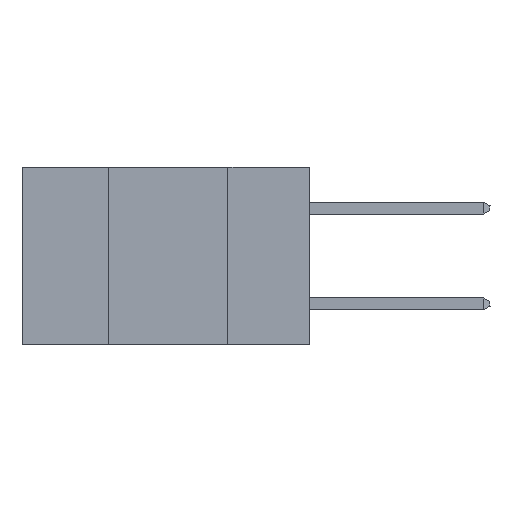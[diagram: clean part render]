
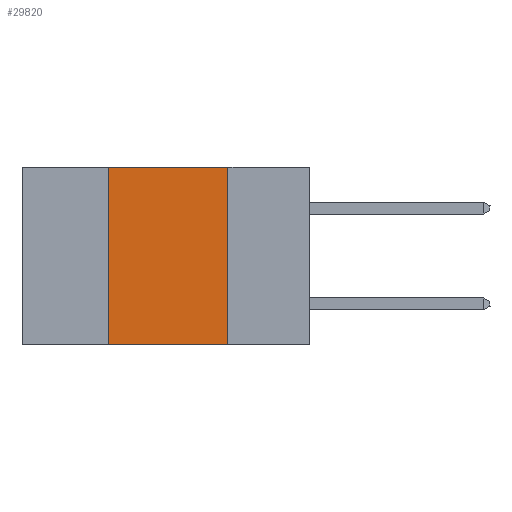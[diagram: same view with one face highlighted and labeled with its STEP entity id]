
A CAD part, left-side view. The second image highlights one B-rep face of the part: STEP entity #29820.
In plain terms, the highlighted planar face has unit normal (-1, 0, 0).
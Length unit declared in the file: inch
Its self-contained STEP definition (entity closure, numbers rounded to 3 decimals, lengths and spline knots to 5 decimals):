
#1232 = ORIENTED_EDGE ( 'NONE', *, *, #31208, .T. ) ;
#1820 = VERTEX_POINT ( 'NONE', #5468 ) ;
#1904 = CARTESIAN_POINT ( 'NONE',  ( 0., 0.17, 0. ) ) ;
#2602 = DIRECTION ( 'NONE',  ( 0., 0., -1. ) ) ;
#3561 = VECTOR ( 'NONE', #22706, 39.37008 ) ;
#4249 = LINE ( 'NONE', #20107, #28811 ) ;
#4279 = LINE ( 'NONE', #24696, #29614 ) ;
#4866 = PLANE ( 'NONE',  #22810 ) ;
#4954 = DIRECTION ( 'NONE',  ( 0., 0., 1. ) ) ;
#5284 = DIRECTION ( 'NONE',  ( 1., 0., 0. ) ) ;
#5468 = CARTESIAN_POINT ( 'NONE',  ( 0., 0.42, -0.37 ) ) ;
#6289 = EDGE_CURVE ( 'NONE', #16522, #19046, #11059, .T. ) ;
#6829 = DIRECTION ( 'NONE',  ( 0., 0., -1. ) ) ;
#7354 = ORIENTED_EDGE ( 'NONE', *, *, #28133, .F. ) ;
#9899 = DIRECTION ( 'NONE',  ( 0., -1., 0. ) ) ;
#11059 = LINE ( 'NONE', #11565, #19908 ) ;
#11565 = CARTESIAN_POINT ( 'NONE',  ( 0., 0.17, 0. ) ) ;
#14730 = LINE ( 'NONE', #27120, #3561 ) ;
#16067 = ORIENTED_EDGE ( 'NONE', *, *, #28015, .F. ) ;
#16522 = VERTEX_POINT ( 'NONE', #1904 ) ;
#19046 = VERTEX_POINT ( 'NONE', #31776 ) ;
#19429 = EDGE_LOOP ( 'NONE', ( #23820, #7354, #16067, #1232 ) ) ;
#19908 = VECTOR ( 'NONE', #6829, 39.37008 ) ;
#20107 = CARTESIAN_POINT ( 'NONE',  ( 0., 0.6, 0. ) ) ;
#22706 = DIRECTION ( 'NONE',  ( 0., -1., 0. ) ) ;
#22810 = AXIS2_PLACEMENT_3D ( 'NONE', #27292, #5284, #2602 ) ;
#22857 = FACE_OUTER_BOUND ( 'NONE', #19429, .T. ) ;
#23820 = ORIENTED_EDGE ( 'NONE', *, *, #6289, .F. ) ;
#24026 = VERTEX_POINT ( 'NONE', #27383 ) ;
#24696 = CARTESIAN_POINT ( 'NONE',  ( 0., 0.42, 0. ) ) ;
#27120 = CARTESIAN_POINT ( 'NONE',  ( 0., 0.6, -0.37 ) ) ;
#27292 = CARTESIAN_POINT ( 'NONE',  ( 0., 0.6, 0. ) ) ;
#27383 = CARTESIAN_POINT ( 'NONE',  ( 0., 0.42, 0. ) ) ;
#28015 = EDGE_CURVE ( 'NONE', #1820, #24026, #4279, .T. ) ;
#28133 = EDGE_CURVE ( 'NONE', #24026, #16522, #4249, .T. ) ;
#28811 = VECTOR ( 'NONE', #9899, 39.37008 ) ;
#29614 = VECTOR ( 'NONE', #4954, 39.37008 ) ;
#29820 = ADVANCED_FACE ( 'NONE', ( #22857 ), #4866, .F. ) ;
#31208 = EDGE_CURVE ( 'NONE', #1820, #19046, #14730, .T. ) ;
#31776 = CARTESIAN_POINT ( 'NONE',  ( 0., 0.17, -0.37 ) ) ;
